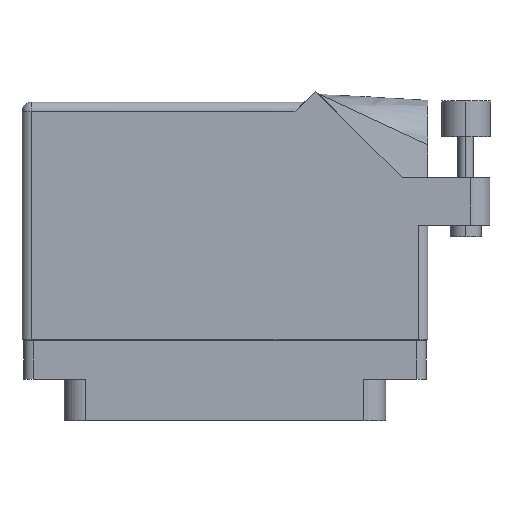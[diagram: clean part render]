
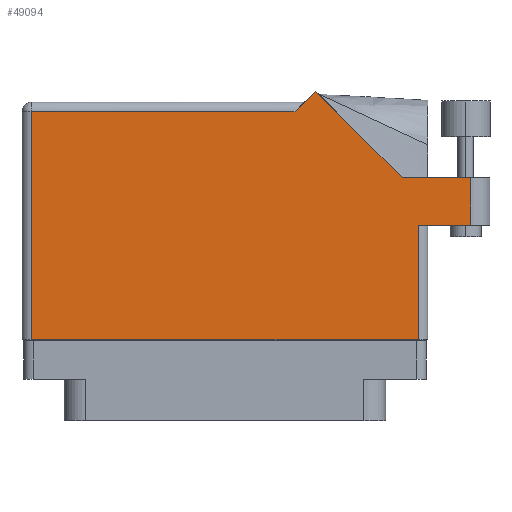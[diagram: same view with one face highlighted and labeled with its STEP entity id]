
A CAD part, front view. The second image highlights one B-rep face of the part: STEP entity #49094.
In plain terms, the highlighted face is planar.
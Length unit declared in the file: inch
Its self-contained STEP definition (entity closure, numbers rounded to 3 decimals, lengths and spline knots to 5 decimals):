
#59 = ORIENTED_EDGE ( 'NONE', *, *, #27562, .T. ) ;
#291 = LINE ( 'NONE', #16343, #2138 ) ;
#2078 = VECTOR ( 'NONE', #45417, 39.37008 ) ;
#2138 = VECTOR ( 'NONE', #16079, 39.37008 ) ;
#2683 = EDGE_CURVE ( 'NONE', #5175, #15977, #6114, .T. ) ;
#4607 = VECTOR ( 'NONE', #7983, 39.37008 ) ;
#5175 = VERTEX_POINT ( 'NONE', #31498 ) ;
#5274 = VERTEX_POINT ( 'NONE', #40928 ) ;
#5649 = CARTESIAN_POINT ( 'NONE',  ( -1.244, 1.368, 0.455 ) ) ;
#5736 = VERTEX_POINT ( 'NONE', #41127 ) ;
#5773 = FACE_OUTER_BOUND ( 'NONE', #10909, .T. ) ;
#6114 = LINE ( 'NONE', #50252, #13114 ) ;
#7194 = EDGE_CURVE ( 'NONE', #5274, #49383, #11187, .T. ) ;
#7953 = ORIENTED_EDGE ( 'NONE', *, *, #44478, .T. ) ;
#7983 = DIRECTION ( 'NONE',  ( 1., 0., 0. ) ) ;
#9427 = EDGE_CURVE ( 'NONE', #15889, #5736, #15884, .T. ) ;
#10109 = VECTOR ( 'NONE', #51905, 39.37008 ) ;
#10326 = EDGE_CURVE ( 'NONE', #5736, #5175, #44873, .T. ) ;
#10796 = VERTEX_POINT ( 'NONE', #18470 ) ;
#10909 = EDGE_LOOP ( 'NONE', ( #50972, #51936, #51495, #46296, #19906, #44165, #59, #28710, #7953 ) ) ;
#11187 = LINE ( 'NONE', #50065, #33763 ) ;
#13114 = VECTOR ( 'NONE', #43601, 39.37008 ) ;
#13449 = VERTEX_POINT ( 'NONE', #30450 ) ;
#13882 = CARTESIAN_POINT ( 'NONE',  ( 1.244, 0.637, 0.455 ) ) ;
#15165 = PLANE ( 'NONE',  #36809 ) ;
#15741 = VERTEX_POINT ( 'NONE', #34326 ) ;
#15884 = LINE ( 'NONE', #27672, #4607 ) ;
#15889 = VERTEX_POINT ( 'NONE', #13882 ) ;
#15977 = VERTEX_POINT ( 'NONE', #50905 ) ;
#16079 = DIRECTION ( 'NONE',  ( 0., -1., 0. ) ) ;
#16343 = CARTESIAN_POINT ( 'NONE',  ( -1.244, -0.1, 0.455 ) ) ;
#16445 = EDGE_CURVE ( 'NONE', #10796, #5274, #47147, .T. ) ;
#17044 = DIRECTION ( 'NONE',  ( 0., 1., 0. ) ) ;
#18470 = CARTESIAN_POINT ( 'NONE',  ( 0.58371, 1.50071, 0.455 ) ) ;
#19063 = CARTESIAN_POINT ( 'NONE',  ( 0.513, 1.43, 0.455 ) ) ;
#19859 = LINE ( 'NONE', #35853, #10109 ) ;
#19906 = ORIENTED_EDGE ( 'NONE', *, *, #16445, .T. ) ;
#21619 = VECTOR ( 'NONE', #35052, 39.37008 ) ;
#26708 = VECTOR ( 'NONE', #17044, 39.37008 ) ;
#26934 = DIRECTION ( 'NONE',  ( -1., 0., 0. ) ) ;
#26964 = CARTESIAN_POINT ( 'NONE',  ( -1.306, 1.43, 0.455 ) ) ;
#27562 = EDGE_CURVE ( 'NONE', #49383, #13449, #291, .T. ) ;
#27672 = CARTESIAN_POINT ( 'NONE',  ( 1.306, 0.637, 0.455 ) ) ;
#28710 = ORIENTED_EDGE ( 'NONE', *, *, #44567, .T. ) ;
#28839 = CARTESIAN_POINT ( 'NONE',  ( 1.581, 0.944, 0.455 ) ) ;
#29392 = CARTESIAN_POINT ( 'NONE',  ( -1.306, -0.1, 0.455 ) ) ;
#29661 = DIRECTION ( 'NONE',  ( -1., 0., 0. ) ) ;
#30450 = CARTESIAN_POINT ( 'NONE',  ( -1.244, -0.1, 0.455 ) ) ;
#31498 = CARTESIAN_POINT ( 'NONE',  ( 1.581, 0.944, 0.455 ) ) ;
#33324 = DIRECTION ( 'NONE',  ( 0., 1., 0. ) ) ;
#33763 = VECTOR ( 'NONE', #26934, 39.37008 ) ;
#34326 = CARTESIAN_POINT ( 'NONE',  ( 1.244, -0.1, 0.455 ) ) ;
#35052 = DIRECTION ( 'NONE',  ( -0.707, -0.707, 0. ) ) ;
#35853 = CARTESIAN_POINT ( 'NONE',  ( 1.14042, 0.944, 0.455 ) ) ;
#36809 = AXIS2_PLACEMENT_3D ( 'NONE', #26964, #37784, #29661 ) ;
#37218 = VECTOR ( 'NONE', #33324, 39.37008 ) ;
#37784 = DIRECTION ( 'NONE',  ( 0., 0., -1. ) ) ;
#38985 = EDGE_CURVE ( 'NONE', #15977, #10796, #19859, .T. ) ;
#40928 = CARTESIAN_POINT ( 'NONE',  ( 0.451, 1.368, 0.455 ) ) ;
#41127 = CARTESIAN_POINT ( 'NONE',  ( 1.581, 0.637, 0.455 ) ) ;
#41215 = CARTESIAN_POINT ( 'NONE',  ( 1.244, 0.637, 0.455 ) ) ;
#41996 = LINE ( 'NONE', #29392, #2078 ) ;
#43601 = DIRECTION ( 'NONE',  ( -1., 0., 0. ) ) ;
#44165 = ORIENTED_EDGE ( 'NONE', *, *, #7194, .T. ) ;
#44478 = EDGE_CURVE ( 'NONE', #15741, #15889, #45678, .T. ) ;
#44567 = EDGE_CURVE ( 'NONE', #13449, #15741, #41996, .T. ) ;
#44873 = LINE ( 'NONE', #28839, #26708 ) ;
#45417 = DIRECTION ( 'NONE',  ( 1., 0., 0. ) ) ;
#45678 = LINE ( 'NONE', #41215, #37218 ) ;
#46296 = ORIENTED_EDGE ( 'NONE', *, *, #38985, .T. ) ;
#47147 = LINE ( 'NONE', #19063, #21619 ) ;
#49094 = ADVANCED_FACE ( 'NONE', ( #5773 ), #15165, .F. ) ;
#49383 = VERTEX_POINT ( 'NONE', #5649 ) ;
#50065 = CARTESIAN_POINT ( 'NONE',  ( -1.306, 1.368, 0.455 ) ) ;
#50252 = CARTESIAN_POINT ( 'NONE',  ( 1.706, 0.944, 0.455 ) ) ;
#50905 = CARTESIAN_POINT ( 'NONE',  ( 1.14042, 0.944, 0.455 ) ) ;
#50972 = ORIENTED_EDGE ( 'NONE', *, *, #9427, .T. ) ;
#51495 = ORIENTED_EDGE ( 'NONE', *, *, #2683, .T. ) ;
#51905 = DIRECTION ( 'NONE',  ( -0.707, 0.707, 0. ) ) ;
#51936 = ORIENTED_EDGE ( 'NONE', *, *, #10326, .T. ) ;
